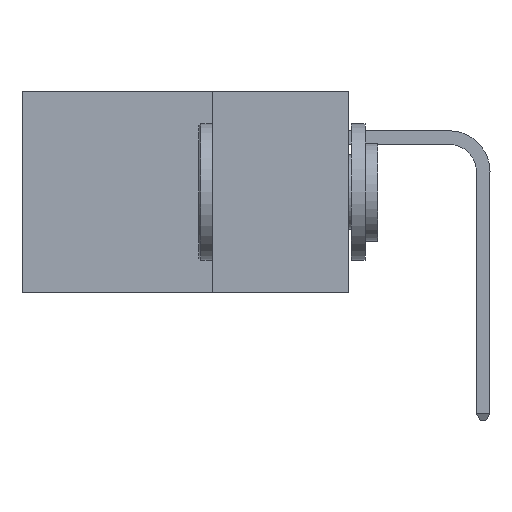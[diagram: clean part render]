
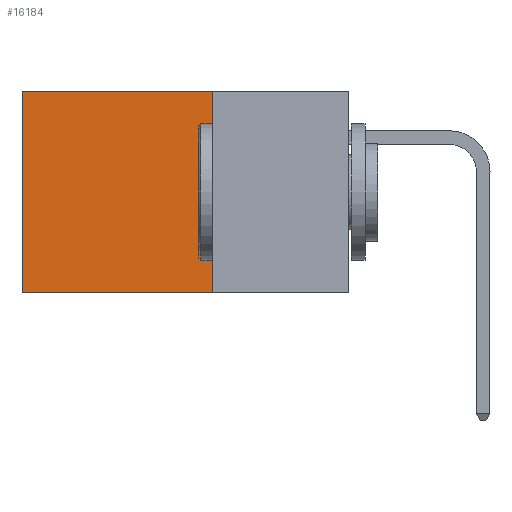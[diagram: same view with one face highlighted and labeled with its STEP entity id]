
A CAD part, left-side view. The second image highlights one B-rep face of the part: STEP entity #16184.
In plain terms, the highlighted planar face has unit normal (-1, 0, 0).
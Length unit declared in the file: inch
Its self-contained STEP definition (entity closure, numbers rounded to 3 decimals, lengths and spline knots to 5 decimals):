
#482 = EDGE_LOOP ( 'NONE', ( #14130, #32762, #6776, #8380 ) ) ;
#1359 = FACE_OUTER_BOUND ( 'NONE', #482, .T. ) ;
#1612 = VERTEX_POINT ( 'NONE', #22251 ) ;
#1974 = EDGE_CURVE ( 'NONE', #19353, #1612, #13327, .T. ) ;
#2991 = CARTESIAN_POINT ( 'NONE',  ( 0.2875, 0.25, -0.37 ) ) ;
#2992 = LINE ( 'NONE', #4919, #13928 ) ;
#3612 = DIRECTION ( 'NONE',  ( 1., 0., 0. ) ) ;
#4919 = CARTESIAN_POINT ( 'NONE',  ( 0.2875, 0.25, -0.37 ) ) ;
#5186 = CARTESIAN_POINT ( 'NONE',  ( 0.2875, 0.25, 0. ) ) ;
#5639 = VERTEX_POINT ( 'NONE', #15411 ) ;
#6359 = CARTESIAN_POINT ( 'NONE',  ( 0.2875, 0.25, 0. ) ) ;
#6776 = ORIENTED_EDGE ( 'NONE', *, *, #22641, .F. ) ;
#7515 = DIRECTION ( 'NONE',  ( 0., 1., 0. ) ) ;
#8380 = ORIENTED_EDGE ( 'NONE', *, *, #1974, .T. ) ;
#10441 = CARTESIAN_POINT ( 'NONE',  ( 0.2875, 0.6, 0. ) ) ;
#10971 = LINE ( 'NONE', #10441, #23921 ) ;
#13226 = DIRECTION ( 'NONE',  ( 0., 0., -1. ) ) ;
#13327 = LINE ( 'NONE', #5186, #29949 ) ;
#13928 = VECTOR ( 'NONE', #7515, 39.37008 ) ;
#14130 = ORIENTED_EDGE ( 'NONE', *, *, #29385, .T. ) ;
#14264 = PLANE ( 'NONE',  #31819 ) ;
#14496 = CARTESIAN_POINT ( 'NONE',  ( 0.2875, 0.25, 0. ) ) ;
#15411 = CARTESIAN_POINT ( 'NONE',  ( 0.2875, 0.6, -0.37 ) ) ;
#16184 = ADVANCED_FACE ( 'NONE', ( #1359 ), #14264, .F. ) ;
#16650 = DIRECTION ( 'NONE',  ( 0., 0., -1. ) ) ;
#17692 = DIRECTION ( 'NONE',  ( 0., 1., 0. ) ) ;
#19353 = VERTEX_POINT ( 'NONE', #31228 ) ;
#20099 = VERTEX_POINT ( 'NONE', #2991 ) ;
#22251 = CARTESIAN_POINT ( 'NONE',  ( 0.2875, 0.6, 0. ) ) ;
#22641 = EDGE_CURVE ( 'NONE', #19353, #20099, #25691, .T. ) ;
#23921 = VECTOR ( 'NONE', #13226, 39.37008 ) ;
#24168 = DIRECTION ( 'NONE',  ( 0., 0., -1. ) ) ;
#25691 = LINE ( 'NONE', #6359, #29762 ) ;
#27782 = EDGE_CURVE ( 'NONE', #20099, #5639, #2992, .T. ) ;
#29385 = EDGE_CURVE ( 'NONE', #1612, #5639, #10971, .T. ) ;
#29762 = VECTOR ( 'NONE', #24168, 39.37008 ) ;
#29949 = VECTOR ( 'NONE', #17692, 39.37008 ) ;
#31228 = CARTESIAN_POINT ( 'NONE',  ( 0.2875, 0.25, 0. ) ) ;
#31819 = AXIS2_PLACEMENT_3D ( 'NONE', #14496, #3612, #16650 ) ;
#32762 = ORIENTED_EDGE ( 'NONE', *, *, #27782, .F. ) ;
